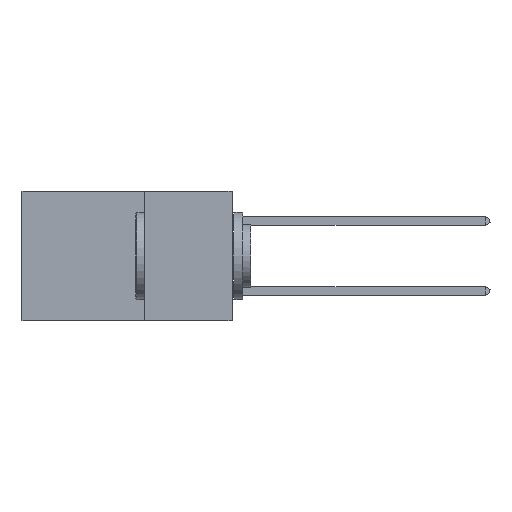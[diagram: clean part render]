
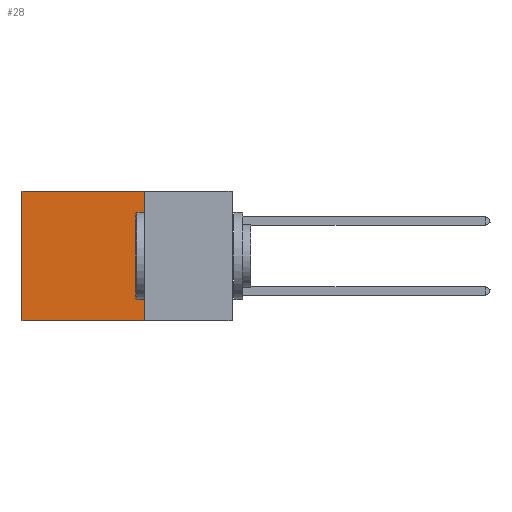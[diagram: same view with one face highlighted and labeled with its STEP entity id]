
A CAD part, left-side view. The second image highlights one B-rep face of the part: STEP entity #28.
In plain terms, the highlighted planar face has unit normal (-1, 0, 0).
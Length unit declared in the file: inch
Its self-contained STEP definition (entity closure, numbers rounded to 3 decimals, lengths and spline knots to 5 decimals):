
#28 = ADVANCED_FACE ( 'NONE', ( #17086 ), #466, .F. ) ;
#355 = CARTESIAN_POINT ( 'NONE',  ( 0.2875, 0.25, 0. ) ) ;
#466 = PLANE ( 'NONE',  #3863 ) ;
#571 = LINE ( 'NONE', #18024, #9874 ) ;
#677 = VERTEX_POINT ( 'NONE', #13693 ) ;
#1193 = VECTOR ( 'NONE', #23207, 39.37008 ) ;
#1425 = EDGE_CURVE ( 'NONE', #2104, #10755, #6776, .T. ) ;
#1476 = CARTESIAN_POINT ( 'NONE',  ( 0.2875, 0.6, 0. ) ) ;
#1593 = LINE ( 'NONE', #10908, #19996 ) ;
#1650 = DIRECTION ( 'NONE',  ( 0., 1., 0. ) ) ;
#2104 = VERTEX_POINT ( 'NONE', #22143 ) ;
#2698 = EDGE_CURVE ( 'NONE', #677, #8825, #9596, .T. ) ;
#2781 = DIRECTION ( 'NONE',  ( 0., 0., -1. ) ) ;
#3863 = AXIS2_PLACEMENT_3D ( 'NONE', #355, #20209, #2781 ) ;
#4981 = ORIENTED_EDGE ( 'NONE', *, *, #1425, .T. ) ;
#5416 = ORIENTED_EDGE ( 'NONE', *, *, #10236, .F. ) ;
#6060 = EDGE_CURVE ( 'NONE', #677, #2104, #571, .T. ) ;
#6776 = LINE ( 'NONE', #1476, #1193 ) ;
#8262 = ORIENTED_EDGE ( 'NONE', *, *, #6060, .T. ) ;
#8825 = VERTEX_POINT ( 'NONE', #12536 ) ;
#8977 = DIRECTION ( 'NONE',  ( 0., 1., 0. ) ) ;
#9596 = LINE ( 'NONE', #12746, #23465 ) ;
#9874 = VECTOR ( 'NONE', #8977, 39.37008 ) ;
#10236 = EDGE_CURVE ( 'NONE', #8825, #10755, #1593, .T. ) ;
#10755 = VERTEX_POINT ( 'NONE', #12218 ) ;
#10908 = CARTESIAN_POINT ( 'NONE',  ( 0.2875, 0.25, -0.37 ) ) ;
#10944 = DIRECTION ( 'NONE',  ( 0., 0., -1. ) ) ;
#12218 = CARTESIAN_POINT ( 'NONE',  ( 0.2875, 0.6, -0.37 ) ) ;
#12536 = CARTESIAN_POINT ( 'NONE',  ( 0.2875, 0.25, -0.37 ) ) ;
#12746 = CARTESIAN_POINT ( 'NONE',  ( 0.2875, 0.25, 0. ) ) ;
#13517 = ORIENTED_EDGE ( 'NONE', *, *, #2698, .F. ) ;
#13693 = CARTESIAN_POINT ( 'NONE',  ( 0.2875, 0.25, 0. ) ) ;
#14508 = EDGE_LOOP ( 'NONE', ( #4981, #5416, #13517, #8262 ) ) ;
#17086 = FACE_OUTER_BOUND ( 'NONE', #14508, .T. ) ;
#18024 = CARTESIAN_POINT ( 'NONE',  ( 0.2875, 0.25, 0. ) ) ;
#19996 = VECTOR ( 'NONE', #1650, 39.37008 ) ;
#20209 = DIRECTION ( 'NONE',  ( 1., 0., 0. ) ) ;
#22143 = CARTESIAN_POINT ( 'NONE',  ( 0.2875, 0.6, 0. ) ) ;
#23207 = DIRECTION ( 'NONE',  ( 0., 0., -1. ) ) ;
#23465 = VECTOR ( 'NONE', #10944, 39.37008 ) ;
